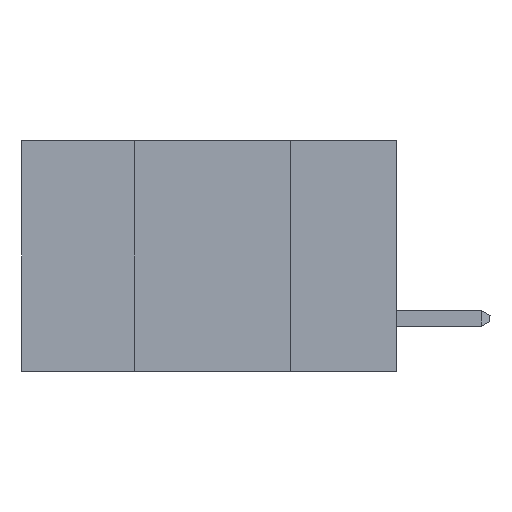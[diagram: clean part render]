
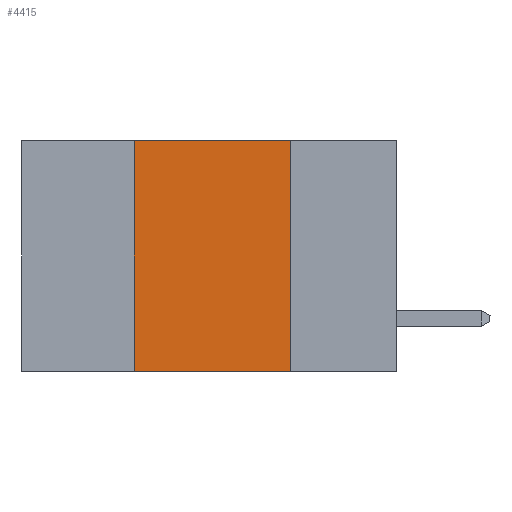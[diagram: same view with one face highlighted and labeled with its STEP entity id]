
A CAD part, left-side view. The second image highlights one B-rep face of the part: STEP entity #4415.
In plain terms, the highlighted planar face has unit normal (-1, 0, 0).
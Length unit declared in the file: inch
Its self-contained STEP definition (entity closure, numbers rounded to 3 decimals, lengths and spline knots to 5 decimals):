
#45 = EDGE_CURVE ( 'NONE', #2067, #6204, #8602, .T. ) ;
#97 = ORIENTED_EDGE ( 'NONE', *, *, #6200, .T. ) ;
#112 = VECTOR ( 'NONE', #4666, 39.37008 ) ;
#874 = CARTESIAN_POINT ( 'NONE',  ( 0., 0.42, 0. ) ) ;
#1110 = AXIS2_PLACEMENT_3D ( 'NONE', #3683, #10241, #7826 ) ;
#1143 = EDGE_CURVE ( 'NONE', #9875, #10334, #2974, .T. ) ;
#1750 = ORIENTED_EDGE ( 'NONE', *, *, #1143, .F. ) ;
#2067 = VERTEX_POINT ( 'NONE', #8223 ) ;
#2115 = PLANE ( 'NONE',  #1110 ) ;
#2479 = DIRECTION ( 'NONE',  ( 0., 0., 1. ) ) ;
#2715 = VECTOR ( 'NONE', #2479, 39.37008 ) ;
#2844 = VECTOR ( 'NONE', #4235, 39.37008 ) ;
#2905 = VECTOR ( 'NONE', #3429, 39.37008 ) ;
#2974 = LINE ( 'NONE', #3416, #2844 ) ;
#3414 = LINE ( 'NONE', #5933, #2905 ) ;
#3416 = CARTESIAN_POINT ( 'NONE',  ( 0., 0.17, 0. ) ) ;
#3429 = DIRECTION ( 'NONE',  ( 0., -1., 0. ) ) ;
#3683 = CARTESIAN_POINT ( 'NONE',  ( 0., 0.6, 0. ) ) ;
#4235 = DIRECTION ( 'NONE',  ( 0., 0., -1. ) ) ;
#4353 = ORIENTED_EDGE ( 'NONE', *, *, #45, .F. ) ;
#4415 = ADVANCED_FACE ( 'NONE', ( #6731 ), #2115, .F. ) ;
#4666 = DIRECTION ( 'NONE',  ( 0., -1., 0. ) ) ;
#5933 = CARTESIAN_POINT ( 'NONE',  ( 0., 0.6, -0.37 ) ) ;
#6200 = EDGE_CURVE ( 'NONE', #2067, #10334, #3414, .T. ) ;
#6204 = VERTEX_POINT ( 'NONE', #7602 ) ;
#6731 = FACE_OUTER_BOUND ( 'NONE', #9687, .T. ) ;
#6803 = LINE ( 'NONE', #7951, #112 ) ;
#7602 = CARTESIAN_POINT ( 'NONE',  ( 0., 0.42, 0. ) ) ;
#7739 = ORIENTED_EDGE ( 'NONE', *, *, #8312, .F. ) ;
#7826 = DIRECTION ( 'NONE',  ( 0., 0., -1. ) ) ;
#7840 = CARTESIAN_POINT ( 'NONE',  ( 0., 0.17, -0.37 ) ) ;
#7951 = CARTESIAN_POINT ( 'NONE',  ( 0., 0.6, 0. ) ) ;
#8223 = CARTESIAN_POINT ( 'NONE',  ( 0., 0.42, -0.37 ) ) ;
#8312 = EDGE_CURVE ( 'NONE', #6204, #9875, #6803, .T. ) ;
#8602 = LINE ( 'NONE', #874, #2715 ) ;
#9328 = CARTESIAN_POINT ( 'NONE',  ( 0., 0.17, 0. ) ) ;
#9687 = EDGE_LOOP ( 'NONE', ( #1750, #7739, #4353, #97 ) ) ;
#9875 = VERTEX_POINT ( 'NONE', #9328 ) ;
#10241 = DIRECTION ( 'NONE',  ( 1., 0., 0. ) ) ;
#10334 = VERTEX_POINT ( 'NONE', #7840 ) ;
